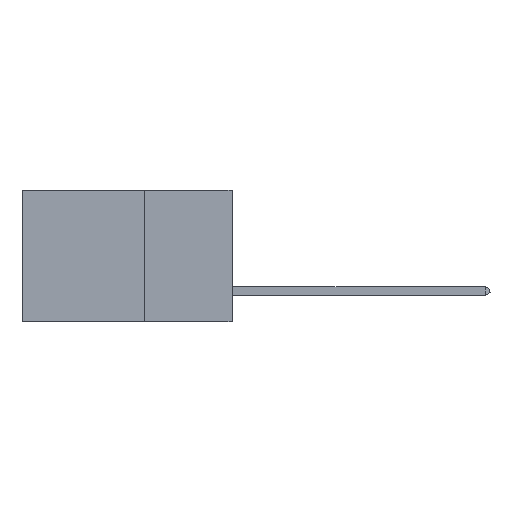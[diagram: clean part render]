
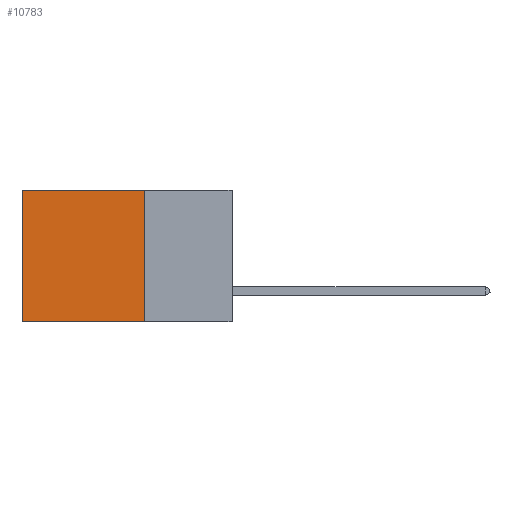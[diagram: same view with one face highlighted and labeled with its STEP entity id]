
A CAD part, left-side view. The second image highlights one B-rep face of the part: STEP entity #10783.
In plain terms, the highlighted planar face has unit normal (-1, 0, 0).
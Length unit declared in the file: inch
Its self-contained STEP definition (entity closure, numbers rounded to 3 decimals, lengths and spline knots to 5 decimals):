
#207 = EDGE_CURVE ( 'NONE', #1227, #3141, #7305, .T. ) ;
#535 = ORIENTED_EDGE ( 'NONE', *, *, #8810, .T. ) ;
#602 = FACE_OUTER_BOUND ( 'NONE', #9768, .T. ) ;
#632 = DIRECTION ( 'NONE',  ( 0., 0., -1. ) ) ;
#1090 = VECTOR ( 'NONE', #13617, 39.37008 ) ;
#1227 = VERTEX_POINT ( 'NONE', #3255 ) ;
#1874 = CARTESIAN_POINT ( 'NONE',  ( 0.2875, 0.25, -0.375 ) ) ;
#2725 = VECTOR ( 'NONE', #632, 39.37008 ) ;
#2733 = ORIENTED_EDGE ( 'NONE', *, *, #11446, .F. ) ;
#2811 = PLANE ( 'NONE',  #7505 ) ;
#3141 = VERTEX_POINT ( 'NONE', #5297 ) ;
#3255 = CARTESIAN_POINT ( 'NONE',  ( 0.2875, 0.25, -0.375 ) ) ;
#4144 = DIRECTION ( 'NONE',  ( 0., 0., -1. ) ) ;
#4692 = EDGE_CURVE ( 'NONE', #8888, #3141, #12612, .T. ) ;
#4871 = LINE ( 'NONE', #9258, #1090 ) ;
#5297 = CARTESIAN_POINT ( 'NONE',  ( 0.2875, 0.6, -0.375 ) ) ;
#5521 = VERTEX_POINT ( 'NONE', #6705 ) ;
#5581 = CARTESIAN_POINT ( 'NONE',  ( 0.2875, 0.25, -0.375 ) ) ;
#6233 = ORIENTED_EDGE ( 'NONE', *, *, #4692, .T. ) ;
#6705 = CARTESIAN_POINT ( 'NONE',  ( 0.2875, 0.25, 0. ) ) ;
#7305 = LINE ( 'NONE', #11690, #9510 ) ;
#7451 = DIRECTION ( 'NONE',  ( 0., 1., 0. ) ) ;
#7505 = AXIS2_PLACEMENT_3D ( 'NONE', #1874, #9415, #12852 ) ;
#7733 = CARTESIAN_POINT ( 'NONE',  ( 0.2875, 0.6, 0. ) ) ;
#8377 = CARTESIAN_POINT ( 'NONE',  ( 0.2875, 0.6, -0.375 ) ) ;
#8583 = ORIENTED_EDGE ( 'NONE', *, *, #207, .F. ) ;
#8810 = EDGE_CURVE ( 'NONE', #5521, #8888, #4871, .T. ) ;
#8888 = VERTEX_POINT ( 'NONE', #7733 ) ;
#9258 = CARTESIAN_POINT ( 'NONE',  ( 0.2875, 0.25, 0. ) ) ;
#9415 = DIRECTION ( 'NONE',  ( 1., 0., 0. ) ) ;
#9510 = VECTOR ( 'NONE', #7451, 39.37008 ) ;
#9768 = EDGE_LOOP ( 'NONE', ( #6233, #8583, #2733, #535 ) ) ;
#10783 = ADVANCED_FACE ( 'NONE', ( #602 ), #2811, .F. ) ;
#11446 = EDGE_CURVE ( 'NONE', #5521, #1227, #11914, .T. ) ;
#11690 = CARTESIAN_POINT ( 'NONE',  ( 0.2875, 0.25, -0.375 ) ) ;
#11914 = LINE ( 'NONE', #5581, #12554 ) ;
#12554 = VECTOR ( 'NONE', #4144, 39.37008 ) ;
#12612 = LINE ( 'NONE', #8377, #2725 ) ;
#12852 = DIRECTION ( 'NONE',  ( 0., 0., -1. ) ) ;
#13617 = DIRECTION ( 'NONE',  ( 0., 1., 0. ) ) ;
